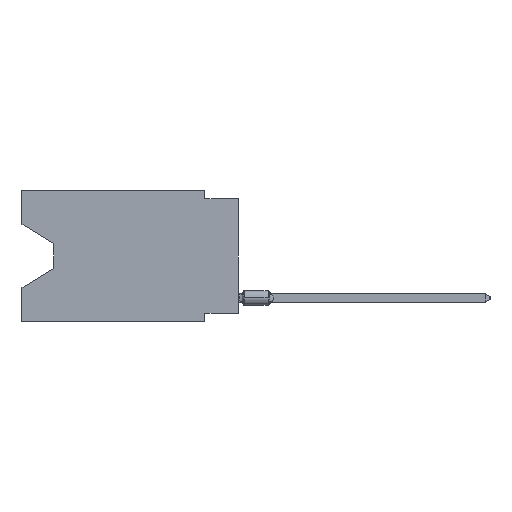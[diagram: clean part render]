
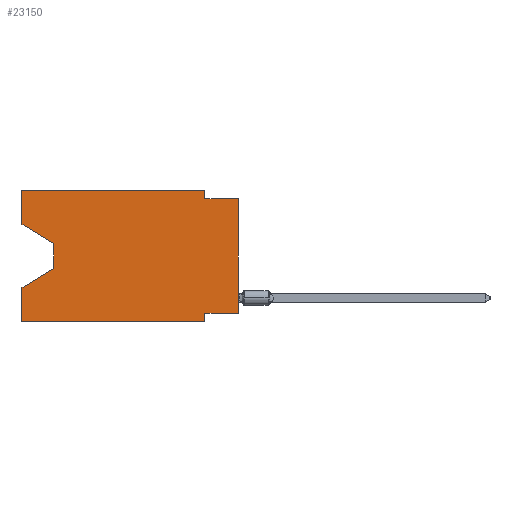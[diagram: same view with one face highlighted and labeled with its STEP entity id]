
A CAD part, left-side view. The second image highlights one B-rep face of the part: STEP entity #23150.
In plain terms, the highlighted planar face has unit normal (-1, 0, 0).
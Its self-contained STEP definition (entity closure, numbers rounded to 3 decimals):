
#268 = VECTOR ( 'NONE', #53373, 1000. ) ;
#392 = CARTESIAN_POINT ( 'NONE',  ( 0., 16.383, -2.546 ) ) ;
#802 = DIRECTION ( 'NONE',  ( 0., 0., 1. ) ) ;
#1074 = EDGE_CURVE ( 'NONE', #27175, #42840, #48731, .T. ) ;
#2287 = VECTOR ( 'NONE', #802, 1000. ) ;
#3149 = EDGE_LOOP ( 'NONE', ( #19528, #9938, #14969, #18141, #16017, #31007, #18782, #18052, #53717, #12431, #3794, #45773 ) ) ;
#3794 = ORIENTED_EDGE ( 'NONE', *, *, #22518, .F. ) ;
#4098 = VECTOR ( 'NONE', #50115, 1000. ) ;
#4299 = DIRECTION ( 'NONE',  ( 0., -1., 0. ) ) ;
#5222 = VERTEX_POINT ( 'NONE', #29053 ) ;
#6810 = VECTOR ( 'NONE', #8570, 1000. ) ;
#6998 = DIRECTION ( 'NONE',  ( 0., 1., 0. ) ) ;
#7021 = VECTOR ( 'NONE', #34113, 1000. ) ;
#7545 = CARTESIAN_POINT ( 'NONE',  ( 0., 0., -9.271 ) ) ;
#8127 = CARTESIAN_POINT ( 'NONE',  ( 0., 0., -0.635 ) ) ;
#8244 = VERTEX_POINT ( 'NONE', #31853 ) ;
#8295 = CARTESIAN_POINT ( 'NONE',  ( 0., 16.383, 0. ) ) ;
#8499 = DIRECTION ( 'NONE',  ( 0., -0.855, -0.519 ) ) ;
#8570 = DIRECTION ( 'NONE',  ( 0., -1., 0. ) ) ;
#9339 = CARTESIAN_POINT ( 'NONE',  ( 0., 13.97, -5.893 ) ) ;
#9644 = VERTEX_POINT ( 'NONE', #33260 ) ;
#9938 = ORIENTED_EDGE ( 'NONE', *, *, #1074, .T. ) ;
#11181 = VERTEX_POINT ( 'NONE', #392 ) ;
#11296 = DIRECTION ( 'NONE',  ( 1., 0., 0. ) ) ;
#12431 = ORIENTED_EDGE ( 'NONE', *, *, #37884, .F. ) ;
#12860 = PLANE ( 'NONE',  #43452 ) ;
#13185 = CARTESIAN_POINT ( 'NONE',  ( 0., 2.54, 0. ) ) ;
#14052 = VERTEX_POINT ( 'NONE', #53609 ) ;
#14969 = ORIENTED_EDGE ( 'NONE', *, *, #16656, .T. ) ;
#16017 = ORIENTED_EDGE ( 'NONE', *, *, #52433, .T. ) ;
#16077 = LINE ( 'NONE', #24249, #4098 ) ;
#16656 = EDGE_CURVE ( 'NONE', #42840, #5222, #18974, .T. ) ;
#17492 = CARTESIAN_POINT ( 'NONE',  ( 0., 16.383, 0. ) ) ;
#18052 = ORIENTED_EDGE ( 'NONE', *, *, #41648, .T. ) ;
#18141 = ORIENTED_EDGE ( 'NONE', *, *, #37128, .F. ) ;
#18504 = LINE ( 'NONE', #7545, #24548 ) ;
#18782 = ORIENTED_EDGE ( 'NONE', *, *, #24856, .F. ) ;
#18974 = LINE ( 'NONE', #48908, #40352 ) ;
#19528 = ORIENTED_EDGE ( 'NONE', *, *, #50850, .T. ) ;
#20294 = DIRECTION ( 'NONE',  ( 0., 0., -1. ) ) ;
#21245 = DIRECTION ( 'NONE',  ( 0., 0., 1. ) ) ;
#21585 = CARTESIAN_POINT ( 'NONE',  ( 0., 16.383, -2.546 ) ) ;
#21749 = EDGE_CURVE ( 'NONE', #14052, #26374, #16077, .T. ) ;
#22518 = EDGE_CURVE ( 'NONE', #48670, #47638, #24129, .T. ) ;
#22918 = LINE ( 'NONE', #17492, #7021 ) ;
#23150 = ADVANCED_FACE ( 'NONE', ( #51660 ), #12860, .F. ) ;
#24129 = LINE ( 'NONE', #8295, #6810 ) ;
#24249 = CARTESIAN_POINT ( 'NONE',  ( 0., 2.54, -9.906 ) ) ;
#24548 = VECTOR ( 'NONE', #6998, 1000. ) ;
#24658 = LINE ( 'NONE', #13185, #34102 ) ;
#24856 = EDGE_CURVE ( 'NONE', #8244, #14052, #18504, .T. ) ;
#26374 = VERTEX_POINT ( 'NONE', #38742 ) ;
#27175 = VERTEX_POINT ( 'NONE', #27856 ) ;
#27722 = EDGE_CURVE ( 'NONE', #9644, #31715, #28321, .T. ) ;
#27856 = CARTESIAN_POINT ( 'NONE',  ( 0., 13.97, -4.013 ) ) ;
#28321 = LINE ( 'NONE', #8127, #52686 ) ;
#29053 = CARTESIAN_POINT ( 'NONE',  ( 0., 16.383, -7.36 ) ) ;
#29341 = VECTOR ( 'NONE', #53195, 1000. ) ;
#29548 = CARTESIAN_POINT ( 'NONE',  ( 0., 16.383, -9.906 ) ) ;
#29709 = LINE ( 'NONE', #50680, #2287 ) ;
#31007 = ORIENTED_EDGE ( 'NONE', *, *, #21749, .F. ) ;
#31715 = VERTEX_POINT ( 'NONE', #38597 ) ;
#31773 = DIRECTION ( 'NONE',  ( 0., 0.855, -0.519 ) ) ;
#31853 = CARTESIAN_POINT ( 'NONE',  ( 0., 0., -9.271 ) ) ;
#33032 = LINE ( 'NONE', #21585, #42733 ) ;
#33260 = CARTESIAN_POINT ( 'NONE',  ( 0., 2.54, -0.635 ) ) ;
#34102 = VECTOR ( 'NONE', #46169, 1000. ) ;
#34113 = DIRECTION ( 'NONE',  ( 0., 0., 1. ) ) ;
#35751 = CARTESIAN_POINT ( 'NONE',  ( 0., 2.54, 0. ) ) ;
#37128 = EDGE_CURVE ( 'NONE', #53429, #5222, #37597, .T. ) ;
#37597 = LINE ( 'NONE', #50377, #46190 ) ;
#37884 = EDGE_CURVE ( 'NONE', #47638, #9644, #24658, .T. ) ;
#38597 = CARTESIAN_POINT ( 'NONE',  ( 0., 0., -0.635 ) ) ;
#38672 = CARTESIAN_POINT ( 'NONE',  ( 0., 16.383, 0. ) ) ;
#38742 = CARTESIAN_POINT ( 'NONE',  ( 0., 2.54, -9.906 ) ) ;
#40352 = VECTOR ( 'NONE', #31773, 1000. ) ;
#40577 = CARTESIAN_POINT ( 'NONE',  ( 0., 13.97, -4.013 ) ) ;
#41648 = EDGE_CURVE ( 'NONE', #8244, #31715, #29709, .T. ) ;
#42733 = VECTOR ( 'NONE', #8499, 1000. ) ;
#42840 = VERTEX_POINT ( 'NONE', #9339 ) ;
#43452 = AXIS2_PLACEMENT_3D ( 'NONE', #44561, #11296, #20294 ) ;
#44494 = LINE ( 'NONE', #44758, #29341 ) ;
#44561 = CARTESIAN_POINT ( 'NONE',  ( 0., 16.383, 0. ) ) ;
#44758 = CARTESIAN_POINT ( 'NONE',  ( 0., 16.383, -9.906 ) ) ;
#45773 = ORIENTED_EDGE ( 'NONE', *, *, #51007, .F. ) ;
#46169 = DIRECTION ( 'NONE',  ( 0., 0., -1. ) ) ;
#46190 = VECTOR ( 'NONE', #21245, 1000. ) ;
#47638 = VERTEX_POINT ( 'NONE', #35751 ) ;
#48670 = VERTEX_POINT ( 'NONE', #38672 ) ;
#48731 = LINE ( 'NONE', #40577, #268 ) ;
#48908 = CARTESIAN_POINT ( 'NONE',  ( 0., 13.97, -5.893 ) ) ;
#50115 = DIRECTION ( 'NONE',  ( 0., 0., -1. ) ) ;
#50377 = CARTESIAN_POINT ( 'NONE',  ( 0., 16.383, 0. ) ) ;
#50680 = CARTESIAN_POINT ( 'NONE',  ( 0., 0., 0. ) ) ;
#50850 = EDGE_CURVE ( 'NONE', #11181, #27175, #33032, .T. ) ;
#51007 = EDGE_CURVE ( 'NONE', #11181, #48670, #22918, .T. ) ;
#51660 = FACE_OUTER_BOUND ( 'NONE', #3149, .T. ) ;
#52433 = EDGE_CURVE ( 'NONE', #53429, #26374, #44494, .T. ) ;
#52686 = VECTOR ( 'NONE', #4299, 1000. ) ;
#53195 = DIRECTION ( 'NONE',  ( 0., -1., 0. ) ) ;
#53373 = DIRECTION ( 'NONE',  ( 0., 0., -1. ) ) ;
#53429 = VERTEX_POINT ( 'NONE', #29548 ) ;
#53609 = CARTESIAN_POINT ( 'NONE',  ( 0., 2.54, -9.271 ) ) ;
#53717 = ORIENTED_EDGE ( 'NONE', *, *, #27722, .F. ) ;
